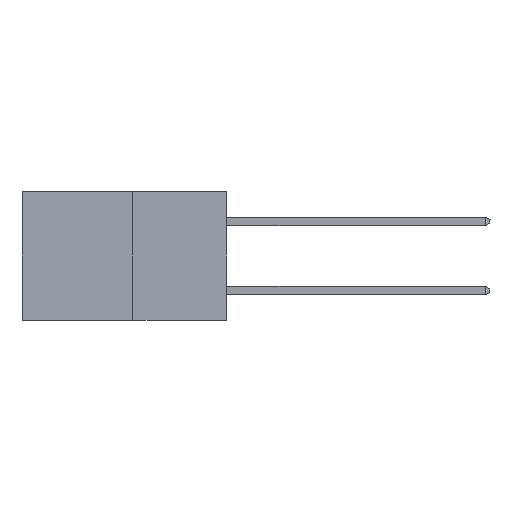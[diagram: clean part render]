
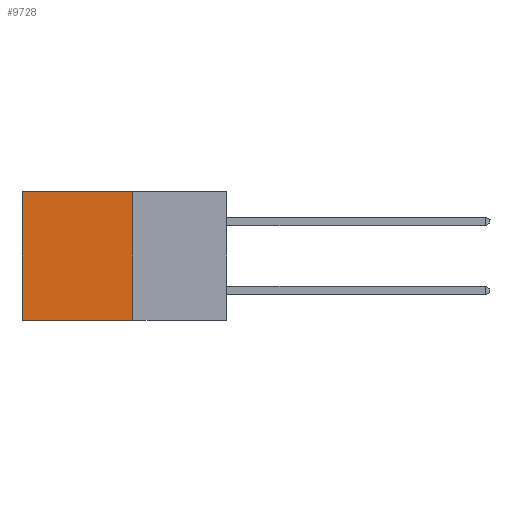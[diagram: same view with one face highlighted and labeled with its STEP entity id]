
A CAD part, left-side view. The second image highlights one B-rep face of the part: STEP entity #9728.
In plain terms, the highlighted planar face has unit normal (-1, 0, 0).
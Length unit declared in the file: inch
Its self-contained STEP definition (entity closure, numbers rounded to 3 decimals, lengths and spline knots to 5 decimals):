
#990 = EDGE_CURVE ( 'NONE', #8567, #8737, #10292, .T. ) ;
#1223 = VECTOR ( 'NONE', #4145, 39.37008 ) ;
#1749 = LINE ( 'NONE', #2055, #14480 ) ;
#1822 = EDGE_CURVE ( 'NONE', #8999, #8894, #1749, .T. ) ;
#1971 = DIRECTION ( 'NONE',  ( 0., 1., 0. ) ) ;
#1973 = AXIS2_PLACEMENT_3D ( 'NONE', #10537, #11721, #4487 ) ;
#2055 = CARTESIAN_POINT ( 'NONE',  ( 0.277, 0.27, 0. ) ) ;
#2268 = ORIENTED_EDGE ( 'NONE', *, *, #11045, .F. ) ;
#2910 = CARTESIAN_POINT ( 'NONE',  ( 0.277, 0.59, -0.37 ) ) ;
#3018 = CARTESIAN_POINT ( 'NONE',  ( 0.277, 0.59, 0. ) ) ;
#3311 = FACE_OUTER_BOUND ( 'NONE', #11349, .T. ) ;
#3857 = DIRECTION ( 'NONE',  ( 0., 0., -1. ) ) ;
#4145 = DIRECTION ( 'NONE',  ( 0., 0., -1. ) ) ;
#4206 = LINE ( 'NONE', #9946, #7037 ) ;
#4487 = DIRECTION ( 'NONE',  ( 0., 0., -1. ) ) ;
#4730 = EDGE_CURVE ( 'NONE', #8894, #8737, #14337, .T. ) ;
#5331 = ORIENTED_EDGE ( 'NONE', *, *, #1822, .T. ) ;
#7037 = VECTOR ( 'NONE', #3857, 39.37008 ) ;
#7051 = VECTOR ( 'NONE', #11829, 39.37008 ) ;
#8567 = VERTEX_POINT ( 'NONE', #10916 ) ;
#8737 = VERTEX_POINT ( 'NONE', #13568 ) ;
#8894 = VERTEX_POINT ( 'NONE', #3018 ) ;
#8999 = VERTEX_POINT ( 'NONE', #10452 ) ;
#9342 = PLANE ( 'NONE',  #1973 ) ;
#9728 = ADVANCED_FACE ( 'NONE', ( #3311 ), #9342, .F. ) ;
#9946 = CARTESIAN_POINT ( 'NONE',  ( 0.277, 0.27, -0.37 ) ) ;
#10292 = LINE ( 'NONE', #15482, #7051 ) ;
#10452 = CARTESIAN_POINT ( 'NONE',  ( 0.277, 0.27, 0. ) ) ;
#10537 = CARTESIAN_POINT ( 'NONE',  ( 0.277, 0.27, -0.37 ) ) ;
#10916 = CARTESIAN_POINT ( 'NONE',  ( 0.277, 0.27, -0.37 ) ) ;
#11045 = EDGE_CURVE ( 'NONE', #8999, #8567, #4206, .T. ) ;
#11349 = EDGE_LOOP ( 'NONE', ( #13981, #12728, #2268, #5331 ) ) ;
#11721 = DIRECTION ( 'NONE',  ( 1., 0., 0. ) ) ;
#11829 = DIRECTION ( 'NONE',  ( 0., 1., 0. ) ) ;
#12728 = ORIENTED_EDGE ( 'NONE', *, *, #990, .F. ) ;
#13568 = CARTESIAN_POINT ( 'NONE',  ( 0.277, 0.59, -0.37 ) ) ;
#13981 = ORIENTED_EDGE ( 'NONE', *, *, #4730, .T. ) ;
#14337 = LINE ( 'NONE', #2910, #1223 ) ;
#14480 = VECTOR ( 'NONE', #1971, 39.37008 ) ;
#15482 = CARTESIAN_POINT ( 'NONE',  ( 0.277, 0.27, -0.37 ) ) ;
